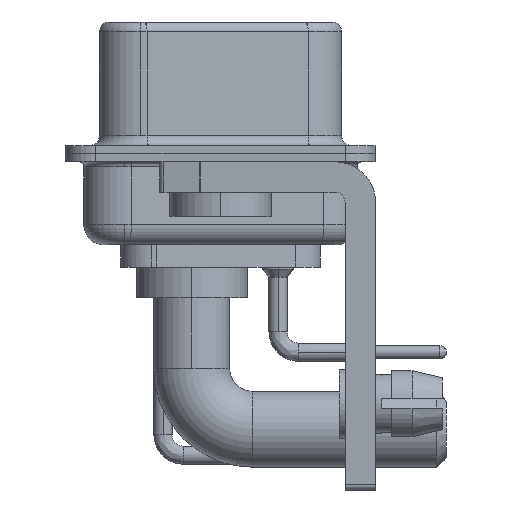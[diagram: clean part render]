
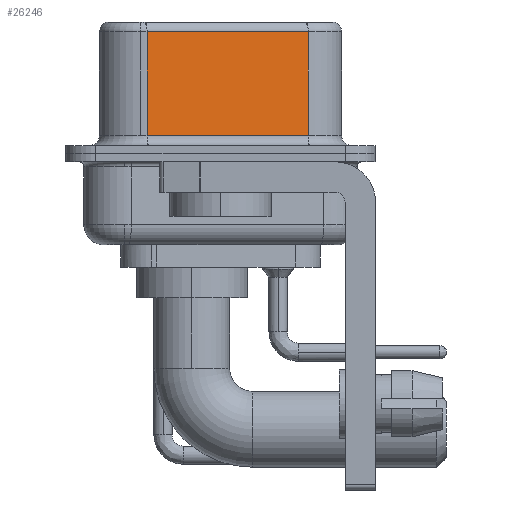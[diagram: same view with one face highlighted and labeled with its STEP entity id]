
A CAD part, left-side view. The second image highlights one B-rep face of the part: STEP entity #26246.
In plain terms, the highlighted planar face has unit normal (-0.985, -0.174, 0).
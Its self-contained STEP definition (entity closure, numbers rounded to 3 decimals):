
#1301 = DIRECTION ( 'NONE',  ( -0.174, 0.985, 0. ) ) ;
#2587 = VECTOR ( 'NONE', #16694, 1000. ) ;
#3546 = CARTESIAN_POINT ( 'NONE',  ( 5.132, -4.322, 6.52 ) ) ;
#3698 = VECTOR ( 'NONE', #21033, 1000. ) ;
#3947 = ORIENTED_EDGE ( 'NONE', *, *, #16768, .F. ) ;
#5261 = CARTESIAN_POINT ( 'NONE',  ( 3.73, 3.628, 6.02 ) ) ;
#7214 = AXIS2_PLACEMENT_3D ( 'NONE', #3546, #21217, #1301 ) ;
#7427 = CARTESIAN_POINT ( 'NONE',  ( 5.132, -4.322, 6.52 ) ) ;
#9364 = CARTESIAN_POINT ( 'NONE',  ( 5.132, -4.322, 0.9 ) ) ;
#11096 = CARTESIAN_POINT ( 'NONE',  ( 3.73, 3.628, 6.52 ) ) ;
#12493 = FACE_OUTER_BOUND ( 'NONE', #20181, .T. ) ;
#12500 = VERTEX_POINT ( 'NONE', #30260 ) ;
#13044 = VERTEX_POINT ( 'NONE', #5261 ) ;
#16089 = EDGE_CURVE ( 'NONE', #12500, #33659, #20899, .T. ) ;
#16099 = ORIENTED_EDGE ( 'NONE', *, *, #31953, .T. ) ;
#16275 = ORIENTED_EDGE ( 'NONE', *, *, #16089, .T. ) ;
#16694 = DIRECTION ( 'NONE',  ( 0., 0., -1. ) ) ;
#16768 = EDGE_CURVE ( 'NONE', #24477, #33659, #21577, .T. ) ;
#17577 = VECTOR ( 'NONE', #30639, 1000. ) ;
#17853 = EDGE_CURVE ( 'NONE', #13044, #12500, #28586, .T. ) ;
#18739 = LINE ( 'NONE', #19307, #17577 ) ;
#19307 = CARTESIAN_POINT ( 'NONE',  ( 5.132, -4.322, 6.02 ) ) ;
#20181 = EDGE_LOOP ( 'NONE', ( #3947, #16099, #20538, #16275 ) ) ;
#20417 = VECTOR ( 'NONE', #29473, 1000. ) ;
#20538 = ORIENTED_EDGE ( 'NONE', *, *, #17853, .T. ) ;
#20899 = LINE ( 'NONE', #34867, #20417 ) ;
#21033 = DIRECTION ( 'NONE',  ( 0., 0., -1. ) ) ;
#21217 = DIRECTION ( 'NONE',  ( 0.985, 0.174, 0. ) ) ;
#21577 = LINE ( 'NONE', #7427, #3698 ) ;
#23490 = PLANE ( 'NONE',  #7214 ) ;
#24477 = VERTEX_POINT ( 'NONE', #30304 ) ;
#26246 = ADVANCED_FACE ( 'NONE', ( #12493 ), #23490, .F. ) ;
#28586 = LINE ( 'NONE', #11096, #2587 ) ;
#29473 = DIRECTION ( 'NONE',  ( 0.174, -0.985, 0. ) ) ;
#30260 = CARTESIAN_POINT ( 'NONE',  ( 3.73, 3.628, 0.9 ) ) ;
#30304 = CARTESIAN_POINT ( 'NONE',  ( 5.132, -4.322, 6.02 ) ) ;
#30639 = DIRECTION ( 'NONE',  ( -0.174, 0.985, 0. ) ) ;
#31953 = EDGE_CURVE ( 'NONE', #24477, #13044, #18739, .T. ) ;
#33659 = VERTEX_POINT ( 'NONE', #9364 ) ;
#34867 = CARTESIAN_POINT ( 'NONE',  ( 5.132, -4.322, 0.9 ) ) ;
